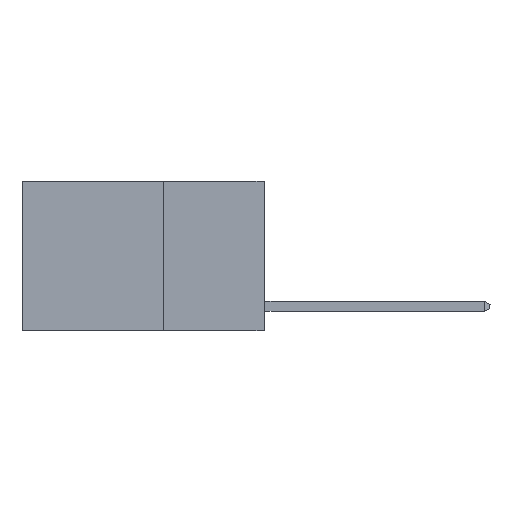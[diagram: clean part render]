
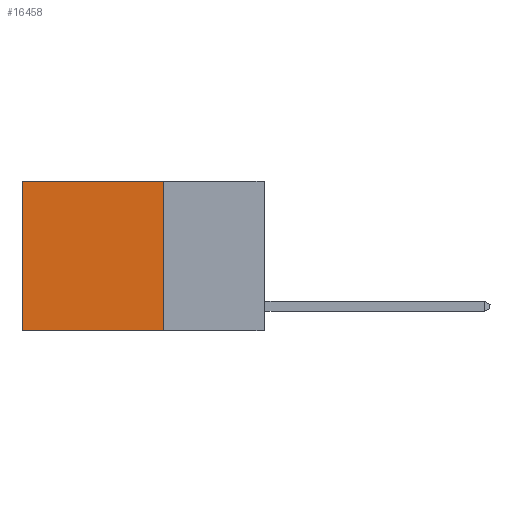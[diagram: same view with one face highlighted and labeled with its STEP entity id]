
A CAD part, left-side view. The second image highlights one B-rep face of the part: STEP entity #16458.
In plain terms, the highlighted planar face has unit normal (-1, 0, 0).
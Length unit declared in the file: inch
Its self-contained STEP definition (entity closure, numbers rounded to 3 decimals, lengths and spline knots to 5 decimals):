
#104 = CARTESIAN_POINT ( 'NONE',  ( 0.2625, 0.25, 0. ) ) ;
#125 = EDGE_CURVE ( 'NONE', #7085, #23542, #20926, .T. ) ;
#359 = ORIENTED_EDGE ( 'NONE', *, *, #125, .F. ) ;
#477 = CARTESIAN_POINT ( 'NONE',  ( 0.2625, 0.25, -0.37 ) ) ;
#1130 = ORIENTED_EDGE ( 'NONE', *, *, #8656, .T. ) ;
#1359 = DIRECTION ( 'NONE',  ( 0., 1., 0. ) ) ;
#1647 = CARTESIAN_POINT ( 'NONE',  ( 0.2625, 0.25, -0.37 ) ) ;
#1655 = LINE ( 'NONE', #20042, #2228 ) ;
#1683 = AXIS2_PLACEMENT_3D ( 'NONE', #19268, #10204, #22927 ) ;
#1876 = LINE ( 'NONE', #104, #20732 ) ;
#2228 = VECTOR ( 'NONE', #7293, 39.37008 ) ;
#3209 = VERTEX_POINT ( 'NONE', #6199 ) ;
#3305 = ORIENTED_EDGE ( 'NONE', *, *, #4185, .F. ) ;
#3390 = CARTESIAN_POINT ( 'NONE',  ( 0.2625, 0.6, 0. ) ) ;
#4185 = EDGE_CURVE ( 'NONE', #3209, #7085, #1876, .T. ) ;
#4712 = PLANE ( 'NONE',  #1683 ) ;
#5450 = EDGE_CURVE ( 'NONE', #8433, #23542, #12124, .T. ) ;
#5695 = DIRECTION ( 'NONE',  ( 0., 0., -1. ) ) ;
#6199 = CARTESIAN_POINT ( 'NONE',  ( 0.2625, 0.25, 0. ) ) ;
#6399 = VECTOR ( 'NONE', #1359, 39.37008 ) ;
#6775 = ORIENTED_EDGE ( 'NONE', *, *, #5450, .T. ) ;
#7085 = VERTEX_POINT ( 'NONE', #477 ) ;
#7265 = VECTOR ( 'NONE', #8916, 39.37008 ) ;
#7293 = DIRECTION ( 'NONE',  ( 0., 1., 0. ) ) ;
#8433 = VERTEX_POINT ( 'NONE', #23069 ) ;
#8656 = EDGE_CURVE ( 'NONE', #3209, #8433, #1655, .T. ) ;
#8916 = DIRECTION ( 'NONE',  ( 0., 0., -1. ) ) ;
#10204 = DIRECTION ( 'NONE',  ( 1., 0., 0. ) ) ;
#12124 = LINE ( 'NONE', #3390, #7265 ) ;
#13629 = EDGE_LOOP ( 'NONE', ( #6775, #359, #3305, #1130 ) ) ;
#15861 = FACE_OUTER_BOUND ( 'NONE', #13629, .T. ) ;
#16458 = ADVANCED_FACE ( 'NONE', ( #15861 ), #4712, .F. ) ;
#19268 = CARTESIAN_POINT ( 'NONE',  ( 0.2625, 0.25, 0. ) ) ;
#20042 = CARTESIAN_POINT ( 'NONE',  ( 0.2625, 0.25, 0. ) ) ;
#20732 = VECTOR ( 'NONE', #5695, 39.37008 ) ;
#20926 = LINE ( 'NONE', #1647, #6399 ) ;
#21607 = CARTESIAN_POINT ( 'NONE',  ( 0.2625, 0.6, -0.37 ) ) ;
#22927 = DIRECTION ( 'NONE',  ( 0., 0., -1. ) ) ;
#23069 = CARTESIAN_POINT ( 'NONE',  ( 0.2625, 0.6, 0. ) ) ;
#23542 = VERTEX_POINT ( 'NONE', #21607 ) ;
